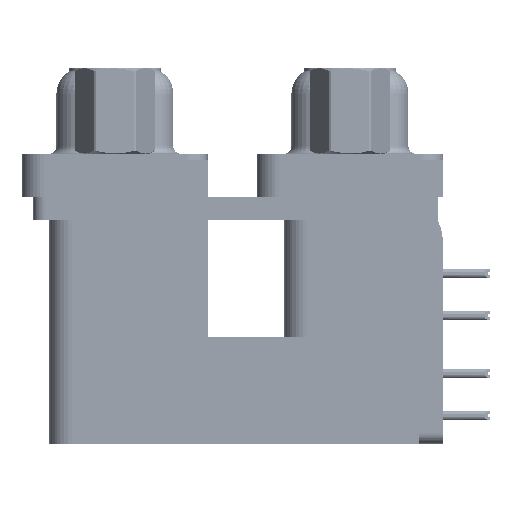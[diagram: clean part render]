
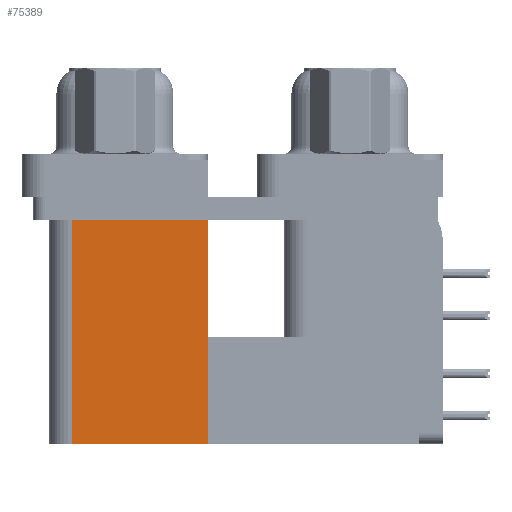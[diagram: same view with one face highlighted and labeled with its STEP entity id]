
A CAD part, left-side view. The second image highlights one B-rep face of the part: STEP entity #75389.
In plain terms, the highlighted planar face has unit normal (-1, 0, 0).
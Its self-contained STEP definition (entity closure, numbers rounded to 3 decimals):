
#428 = VECTOR ( 'NONE', #62315, 1000. ) ;
#3079 = ORIENTED_EDGE ( 'NONE', *, *, #50264, .T. ) ;
#9274 = CARTESIAN_POINT ( 'NONE',  ( 3.79, 18.8, -19.2 ) ) ;
#10841 = CARTESIAN_POINT ( 'NONE',  ( 3.79, 18.8, -19.2 ) ) ;
#11173 = EDGE_CURVE ( 'NONE', #74364, #23134, #61922, .T. ) ;
#15783 = LINE ( 'NONE', #28981, #61964 ) ;
#16247 = EDGE_LOOP ( 'NONE', ( #3079, #42898, #29506, #23047 ) ) ;
#16973 = DIRECTION ( 'NONE',  ( 0., 1., 0. ) ) ;
#19798 = VERTEX_POINT ( 'NONE', #10841 ) ;
#19950 = AXIS2_PLACEMENT_3D ( 'NONE', #57707, #57308, #45699 ) ;
#20527 = LINE ( 'NONE', #9274, #23773 ) ;
#21076 = CARTESIAN_POINT ( 'NONE',  ( 3.79, 18.8, -2.5 ) ) ;
#23047 = ORIENTED_EDGE ( 'NONE', *, *, #11173, .T. ) ;
#23134 = VERTEX_POINT ( 'NONE', #66177 ) ;
#23773 = VECTOR ( 'NONE', #58225, 1000. ) ;
#25270 = VECTOR ( 'NONE', #75726, 1000. ) ;
#28981 = CARTESIAN_POINT ( 'NONE',  ( 3.79, 9.6, -2.5 ) ) ;
#29193 = EDGE_CURVE ( 'NONE', #19798, #59160, #20527, .T. ) ;
#29506 = ORIENTED_EDGE ( 'NONE', *, *, #31464, .F. ) ;
#31464 = EDGE_CURVE ( 'NONE', #74364, #19798, #38829, .T. ) ;
#32814 = FACE_OUTER_BOUND ( 'NONE', #16247, .T. ) ;
#33220 = PLANE ( 'NONE',  #19950 ) ;
#38829 = LINE ( 'NONE', #63285, #25270 ) ;
#42898 = ORIENTED_EDGE ( 'NONE', *, *, #29193, .F. ) ;
#45699 = DIRECTION ( 'NONE',  ( 0., 0., -1. ) ) ;
#50264 = EDGE_CURVE ( 'NONE', #23134, #59160, #15783, .T. ) ;
#57308 = DIRECTION ( 'NONE',  ( 1., 0., 0. ) ) ;
#57707 = CARTESIAN_POINT ( 'NONE',  ( 3.79, 9.6, -19.2 ) ) ;
#58225 = DIRECTION ( 'NONE',  ( 0., 0., 1. ) ) ;
#59160 = VERTEX_POINT ( 'NONE', #21076 ) ;
#61922 = LINE ( 'NONE', #68335, #428 ) ;
#61964 = VECTOR ( 'NONE', #16973, 1000. ) ;
#62315 = DIRECTION ( 'NONE',  ( 0., 0., 1. ) ) ;
#63285 = CARTESIAN_POINT ( 'NONE',  ( 3.79, 9.6, -19.2 ) ) ;
#66177 = CARTESIAN_POINT ( 'NONE',  ( 3.79, 9.6, -2.5 ) ) ;
#68335 = CARTESIAN_POINT ( 'NONE',  ( 3.79, 9.6, -19.2 ) ) ;
#69524 = CARTESIAN_POINT ( 'NONE',  ( 3.79, 9.6, -19.2 ) ) ;
#74364 = VERTEX_POINT ( 'NONE', #69524 ) ;
#75389 = ADVANCED_FACE ( 'NONE', ( #32814 ), #33220, .F. ) ;
#75726 = DIRECTION ( 'NONE',  ( 0., 1., 0. ) ) ;
